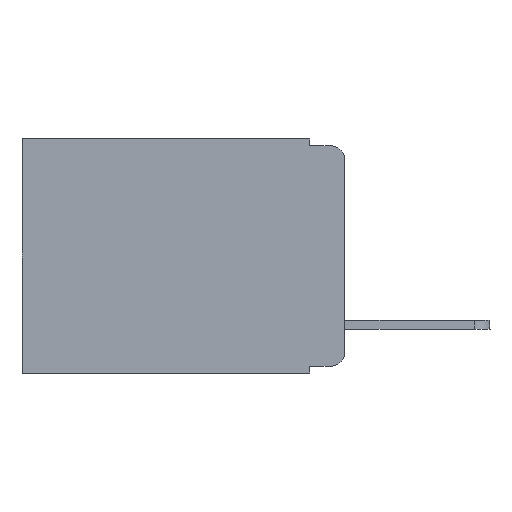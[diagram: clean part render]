
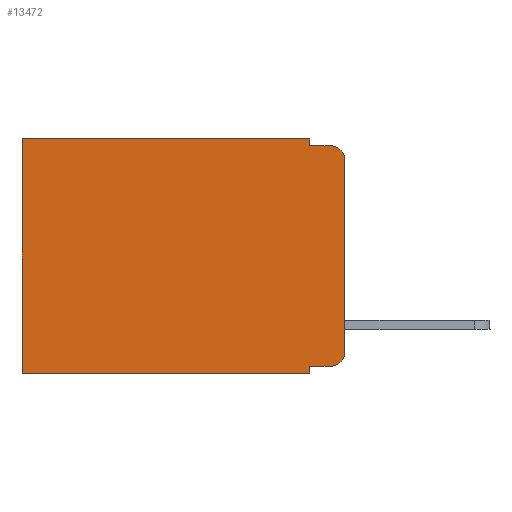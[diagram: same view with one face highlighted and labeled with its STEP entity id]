
A CAD part, left-side view. The second image highlights one B-rep face of the part: STEP entity #13472.
In plain terms, the highlighted planar face has unit normal (-1, 0, 0).
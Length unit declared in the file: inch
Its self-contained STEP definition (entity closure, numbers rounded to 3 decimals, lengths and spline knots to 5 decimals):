
#46 = CARTESIAN_POINT ( 'NONE',  ( 0.298, 0.02, -0.313 ) ) ;
#786 = CARTESIAN_POINT ( 'NONE',  ( 0.298, 0.02, -0.03 ) ) ;
#1070 = VECTOR ( 'NONE', #10719, 39.37008 ) ;
#1395 = AXIS2_PLACEMENT_3D ( 'NONE', #11514, #4437, #9125 ) ;
#1409 = EDGE_LOOP ( 'NONE', ( #9427, #8649, #13176, #5262, #13455, #9262, #5331, #10235, #6896, #13161 ) ) ;
#1466 = CIRCLE ( 'NONE', #6622, 0.02 ) ;
#2049 = EDGE_CURVE ( 'NONE', #12038, #8563, #9600, .T. ) ;
#2111 = VERTEX_POINT ( 'NONE', #6079 ) ;
#2118 = DIRECTION ( 'NONE',  ( 0., 1., 0. ) ) ;
#2264 = CARTESIAN_POINT ( 'NONE',  ( 0.298, 0.473, 0. ) ) ;
#2578 = EDGE_CURVE ( 'NONE', #8276, #11182, #2736, .T. ) ;
#2736 = LINE ( 'NONE', #5339, #14945 ) ;
#3061 = EDGE_CURVE ( 'NONE', #6554, #8563, #1466, .T. ) ;
#3262 = AXIS2_PLACEMENT_3D ( 'NONE', #46, #10722, #14102 ) ;
#3266 = CARTESIAN_POINT ( 'NONE',  ( 0.298, 0., -0.313 ) ) ;
#3344 = CARTESIAN_POINT ( 'NONE',  ( 0.298, 0., -0.03 ) ) ;
#3521 = VECTOR ( 'NONE', #2118, 39.37008 ) ;
#3548 = DIRECTION ( 'NONE',  ( 0., 0., -1. ) ) ;
#3561 = CARTESIAN_POINT ( 'NONE',  ( 0.298, 0.473, -0.343 ) ) ;
#4353 = LINE ( 'NONE', #8774, #9417 ) ;
#4437 = DIRECTION ( 'NONE',  ( 1., 0., 0. ) ) ;
#4639 = EDGE_CURVE ( 'NONE', #6554, #10628, #9291, .T. ) ;
#4677 = VERTEX_POINT ( 'NONE', #9515 ) ;
#5122 = LINE ( 'NONE', #11031, #5724 ) ;
#5262 = ORIENTED_EDGE ( 'NONE', *, *, #11702, .F. ) ;
#5331 = ORIENTED_EDGE ( 'NONE', *, *, #2578, .F. ) ;
#5339 = CARTESIAN_POINT ( 'NONE',  ( 0.298, 0., -0.343 ) ) ;
#5606 = FACE_OUTER_BOUND ( 'NONE', #1409, .T. ) ;
#5724 = VECTOR ( 'NONE', #14469, 39.37008 ) ;
#6079 = CARTESIAN_POINT ( 'NONE',  ( 0.298, 0.02, -0.333 ) ) ;
#6141 = EDGE_CURVE ( 'NONE', #4677, #8276, #4353, .T. ) ;
#6554 = VERTEX_POINT ( 'NONE', #3344 ) ;
#6622 = AXIS2_PLACEMENT_3D ( 'NONE', #786, #13599, #11464 ) ;
#6694 = VERTEX_POINT ( 'NONE', #2264 ) ;
#6896 = ORIENTED_EDGE ( 'NONE', *, *, #8991, .T. ) ;
#7019 = LINE ( 'NONE', #11681, #8229 ) ;
#7221 = LINE ( 'NONE', #12865, #1070 ) ;
#7439 = DIRECTION ( 'NONE',  ( 0., 1., 0. ) ) ;
#7634 = CARTESIAN_POINT ( 'NONE',  ( 0.298, 0.051, -0.343 ) ) ;
#8023 = VERTEX_POINT ( 'NONE', #11467 ) ;
#8229 = VECTOR ( 'NONE', #3548, 39.37008 ) ;
#8276 = VERTEX_POINT ( 'NONE', #7634 ) ;
#8563 = VERTEX_POINT ( 'NONE', #10662 ) ;
#8649 = ORIENTED_EDGE ( 'NONE', *, *, #3061, .T. ) ;
#8774 = CARTESIAN_POINT ( 'NONE',  ( 0.298, 0.051, 0. ) ) ;
#8991 = EDGE_CURVE ( 'NONE', #4677, #2111, #7221, .T. ) ;
#9125 = DIRECTION ( 'NONE',  ( 0., 0., -1. ) ) ;
#9262 = ORIENTED_EDGE ( 'NONE', *, *, #11490, .T. ) ;
#9291 = LINE ( 'NONE', #11970, #13779 ) ;
#9417 = VECTOR ( 'NONE', #15085, 39.37008 ) ;
#9427 = ORIENTED_EDGE ( 'NONE', *, *, #4639, .F. ) ;
#9515 = CARTESIAN_POINT ( 'NONE',  ( 0.298, 0.051, -0.333 ) ) ;
#9600 = LINE ( 'NONE', #13205, #13457 ) ;
#9882 = CIRCLE ( 'NONE', #3262, 0.02 ) ;
#10235 = ORIENTED_EDGE ( 'NONE', *, *, #6141, .F. ) ;
#10271 = PLANE ( 'NONE',  #1395 ) ;
#10317 = CARTESIAN_POINT ( 'NONE',  ( 0.298, 0., 0. ) ) ;
#10341 = EDGE_CURVE ( 'NONE', #2111, #10628, #9882, .T. ) ;
#10627 = EDGE_CURVE ( 'NONE', #8023, #6694, #14919, .T. ) ;
#10628 = VERTEX_POINT ( 'NONE', #3266 ) ;
#10662 = CARTESIAN_POINT ( 'NONE',  ( 0.298, 0.02, -0.01 ) ) ;
#10719 = DIRECTION ( 'NONE',  ( 0., -1., 0. ) ) ;
#10722 = DIRECTION ( 'NONE',  ( -1., 0., 0. ) ) ;
#11031 = CARTESIAN_POINT ( 'NONE',  ( 0.298, 0.051, 0. ) ) ;
#11182 = VERTEX_POINT ( 'NONE', #3561 ) ;
#11464 = DIRECTION ( 'NONE',  ( 0., 0., -1. ) ) ;
#11467 = CARTESIAN_POINT ( 'NONE',  ( 0.298, 0.051, 0. ) ) ;
#11490 = EDGE_CURVE ( 'NONE', #6694, #11182, #7019, .T. ) ;
#11514 = CARTESIAN_POINT ( 'NONE',  ( 0.298, 0., 0. ) ) ;
#11681 = CARTESIAN_POINT ( 'NONE',  ( 0.298, 0.473, 0. ) ) ;
#11702 = EDGE_CURVE ( 'NONE', #8023, #12038, #5122, .T. ) ;
#11970 = CARTESIAN_POINT ( 'NONE',  ( 0.298, 0., 0. ) ) ;
#12038 = VERTEX_POINT ( 'NONE', #13571 ) ;
#12865 = CARTESIAN_POINT ( 'NONE',  ( 0.298, 0.051, -0.333 ) ) ;
#13133 = DIRECTION ( 'NONE',  ( 0., -1., 0. ) ) ;
#13161 = ORIENTED_EDGE ( 'NONE', *, *, #10341, .T. ) ;
#13176 = ORIENTED_EDGE ( 'NONE', *, *, #2049, .F. ) ;
#13205 = CARTESIAN_POINT ( 'NONE',  ( 0.298, 0.051, -0.01 ) ) ;
#13455 = ORIENTED_EDGE ( 'NONE', *, *, #10627, .T. ) ;
#13457 = VECTOR ( 'NONE', #13133, 39.37008 ) ;
#13472 = ADVANCED_FACE ( 'NONE', ( #5606 ), #10271, .F. ) ;
#13571 = CARTESIAN_POINT ( 'NONE',  ( 0.298, 0.051, -0.01 ) ) ;
#13599 = DIRECTION ( 'NONE',  ( -1., 0., 0. ) ) ;
#13779 = VECTOR ( 'NONE', #14113, 39.37008 ) ;
#14102 = DIRECTION ( 'NONE',  ( 0., 0., -1. ) ) ;
#14113 = DIRECTION ( 'NONE',  ( 0., 0., -1. ) ) ;
#14469 = DIRECTION ( 'NONE',  ( 0., 0., -1. ) ) ;
#14919 = LINE ( 'NONE', #10317, #3521 ) ;
#14945 = VECTOR ( 'NONE', #7439, 39.37008 ) ;
#15085 = DIRECTION ( 'NONE',  ( 0., 0., -1. ) ) ;
